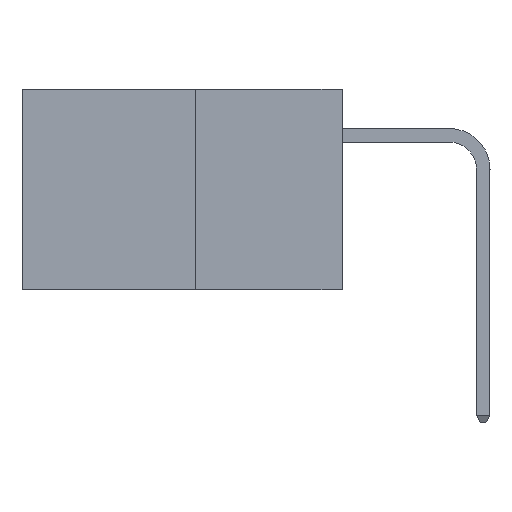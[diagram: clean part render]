
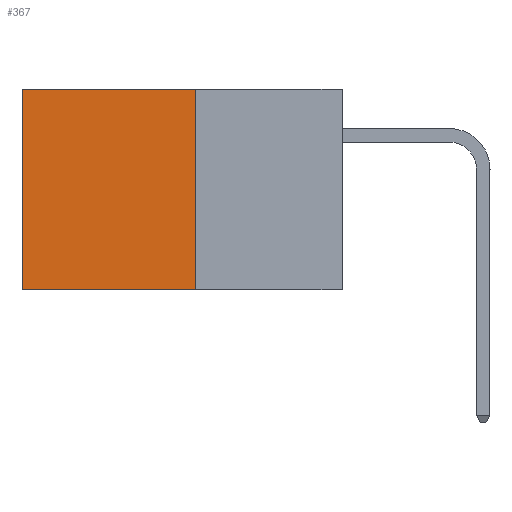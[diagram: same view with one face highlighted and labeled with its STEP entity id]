
A CAD part, left-side view. The second image highlights one B-rep face of the part: STEP entity #367.
In plain terms, the highlighted planar face has unit normal (-1, 0, 0).
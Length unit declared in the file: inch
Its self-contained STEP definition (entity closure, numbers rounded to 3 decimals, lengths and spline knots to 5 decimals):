
#367 = ADVANCED_FACE ( 'NONE', ( #8801 ), #9178, .F. ) ;
#1384 = VECTOR ( 'NONE', #2543, 39.37008 ) ;
#2092 = ORIENTED_EDGE ( 'NONE', *, *, #14246, .T. ) ;
#2162 = VERTEX_POINT ( 'NONE', #17974 ) ;
#2200 = AXIS2_PLACEMENT_3D ( 'NONE', #14328, #16112, #18639 ) ;
#2543 = DIRECTION ( 'NONE',  ( 0., 0., -1. ) ) ;
#2588 = CARTESIAN_POINT ( 'NONE',  ( 0.277, 0.27, -0.37 ) ) ;
#4186 = VERTEX_POINT ( 'NONE', #10388 ) ;
#4637 = VECTOR ( 'NONE', #17761, 39.37008 ) ;
#5412 = EDGE_CURVE ( 'NONE', #14993, #4186, #15511, .T. ) ;
#6029 = VECTOR ( 'NONE', #13316, 39.37008 ) ;
#7898 = VERTEX_POINT ( 'NONE', #13962 ) ;
#8801 = FACE_OUTER_BOUND ( 'NONE', #18235, .T. ) ;
#9178 = PLANE ( 'NONE',  #2200 ) ;
#9862 = EDGE_CURVE ( 'NONE', #4186, #2162, #12259, .T. ) ;
#10388 = CARTESIAN_POINT ( 'NONE',  ( 0.277, 0.27, -0.37 ) ) ;
#10993 = ORIENTED_EDGE ( 'NONE', *, *, #9862, .F. ) ;
#11688 = EDGE_CURVE ( 'NONE', #7898, #2162, #17470, .T. ) ;
#11864 = CARTESIAN_POINT ( 'NONE',  ( 0.277, 0.59, -0.37 ) ) ;
#12259 = LINE ( 'NONE', #16931, #4637 ) ;
#12812 = ORIENTED_EDGE ( 'NONE', *, *, #11688, .T. ) ;
#12871 = VECTOR ( 'NONE', #16266, 39.37008 ) ;
#13302 = LINE ( 'NONE', #16210, #12871 ) ;
#13316 = DIRECTION ( 'NONE',  ( 0., 0., -1. ) ) ;
#13962 = CARTESIAN_POINT ( 'NONE',  ( 0.277, 0.59, 0. ) ) ;
#14246 = EDGE_CURVE ( 'NONE', #14993, #7898, #13302, .T. ) ;
#14328 = CARTESIAN_POINT ( 'NONE',  ( 0.277, 0.27, -0.37 ) ) ;
#14993 = VERTEX_POINT ( 'NONE', #16307 ) ;
#15511 = LINE ( 'NONE', #2588, #1384 ) ;
#16112 = DIRECTION ( 'NONE',  ( 1., 0., 0. ) ) ;
#16210 = CARTESIAN_POINT ( 'NONE',  ( 0.277, 0.27, 0. ) ) ;
#16266 = DIRECTION ( 'NONE',  ( 0., 1., 0. ) ) ;
#16307 = CARTESIAN_POINT ( 'NONE',  ( 0.277, 0.27, 0. ) ) ;
#16931 = CARTESIAN_POINT ( 'NONE',  ( 0.277, 0.27, -0.37 ) ) ;
#17112 = ORIENTED_EDGE ( 'NONE', *, *, #5412, .F. ) ;
#17470 = LINE ( 'NONE', #11864, #6029 ) ;
#17761 = DIRECTION ( 'NONE',  ( 0., 1., 0. ) ) ;
#17974 = CARTESIAN_POINT ( 'NONE',  ( 0.277, 0.59, -0.37 ) ) ;
#18235 = EDGE_LOOP ( 'NONE', ( #12812, #10993, #17112, #2092 ) ) ;
#18639 = DIRECTION ( 'NONE',  ( 0., 0., -1. ) ) ;
